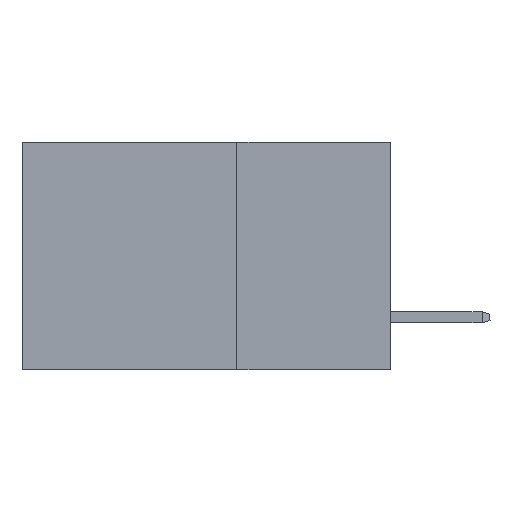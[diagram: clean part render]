
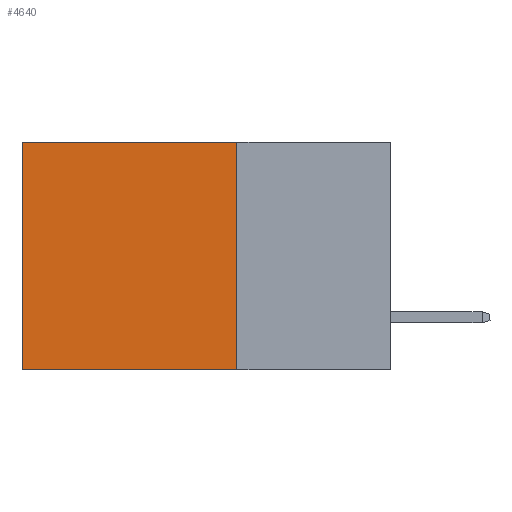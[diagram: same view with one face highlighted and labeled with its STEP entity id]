
A CAD part, left-side view. The second image highlights one B-rep face of the part: STEP entity #4640.
In plain terms, the highlighted planar face has unit normal (-1, 0, 0).
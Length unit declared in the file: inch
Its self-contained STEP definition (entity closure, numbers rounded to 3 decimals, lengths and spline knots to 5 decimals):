
#786 = EDGE_LOOP ( 'NONE', ( #9235, #7932, #9118, #1671 ) ) ;
#1007 = FACE_OUTER_BOUND ( 'NONE', #786, .T. ) ;
#1011 = DIRECTION ( 'NONE',  ( 0., 0., -1. ) ) ;
#1671 = ORIENTED_EDGE ( 'NONE', *, *, #9605, .T. ) ;
#1731 = CARTESIAN_POINT ( 'NONE',  ( 0.2875, 0.25, -0.37 ) ) ;
#1818 = DIRECTION ( 'NONE',  ( 0., 1., 0. ) ) ;
#2927 = VERTEX_POINT ( 'NONE', #9430 ) ;
#2957 = VERTEX_POINT ( 'NONE', #1731 ) ;
#3321 = DIRECTION ( 'NONE',  ( 0., 1., 0. ) ) ;
#3381 = CARTESIAN_POINT ( 'NONE',  ( 0.2875, 0.25, 0. ) ) ;
#3422 = DIRECTION ( 'NONE',  ( 0., 0., -1. ) ) ;
#3686 = AXIS2_PLACEMENT_3D ( 'NONE', #5609, #5507, #3963 ) ;
#3963 = DIRECTION ( 'NONE',  ( 0., 0., -1. ) ) ;
#4066 = PLANE ( 'NONE',  #3686 ) ;
#4213 = CARTESIAN_POINT ( 'NONE',  ( 0.2875, 0.25, -0.37 ) ) ;
#4640 = ADVANCED_FACE ( 'NONE', ( #1007 ), #4066, .F. ) ;
#4786 = VECTOR ( 'NONE', #3422, 39.37008 ) ;
#5059 = VERTEX_POINT ( 'NONE', #9159 ) ;
#5077 = LINE ( 'NONE', #4213, #7218 ) ;
#5281 = LINE ( 'NONE', #8097, #4786 ) ;
#5507 = DIRECTION ( 'NONE',  ( 1., 0., 0. ) ) ;
#5609 = CARTESIAN_POINT ( 'NONE',  ( 0.2875, 0.25, 0. ) ) ;
#5633 = VERTEX_POINT ( 'NONE', #7465 ) ;
#5661 = CARTESIAN_POINT ( 'NONE',  ( 0.2875, 0.25, 0. ) ) ;
#7030 = VECTOR ( 'NONE', #3321, 39.37008 ) ;
#7106 = VECTOR ( 'NONE', #1011, 39.37008 ) ;
#7118 = EDGE_CURVE ( 'NONE', #2927, #2957, #8701, .T. ) ;
#7131 = EDGE_CURVE ( 'NONE', #2957, #5633, #5077, .T. ) ;
#7218 = VECTOR ( 'NONE', #1818, 39.37008 ) ;
#7465 = CARTESIAN_POINT ( 'NONE',  ( 0.2875, 0.6, -0.37 ) ) ;
#7796 = EDGE_CURVE ( 'NONE', #5059, #5633, #5281, .T. ) ;
#7883 = LINE ( 'NONE', #3381, #7030 ) ;
#7932 = ORIENTED_EDGE ( 'NONE', *, *, #7131, .F. ) ;
#8097 = CARTESIAN_POINT ( 'NONE',  ( 0.2875, 0.6, 0. ) ) ;
#8701 = LINE ( 'NONE', #5661, #7106 ) ;
#9118 = ORIENTED_EDGE ( 'NONE', *, *, #7118, .F. ) ;
#9159 = CARTESIAN_POINT ( 'NONE',  ( 0.2875, 0.6, 0. ) ) ;
#9235 = ORIENTED_EDGE ( 'NONE', *, *, #7796, .T. ) ;
#9430 = CARTESIAN_POINT ( 'NONE',  ( 0.2875, 0.25, 0. ) ) ;
#9605 = EDGE_CURVE ( 'NONE', #2927, #5059, #7883, .T. ) ;
